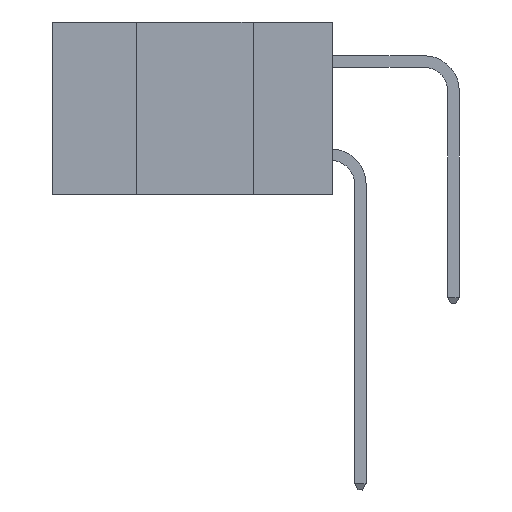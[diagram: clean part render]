
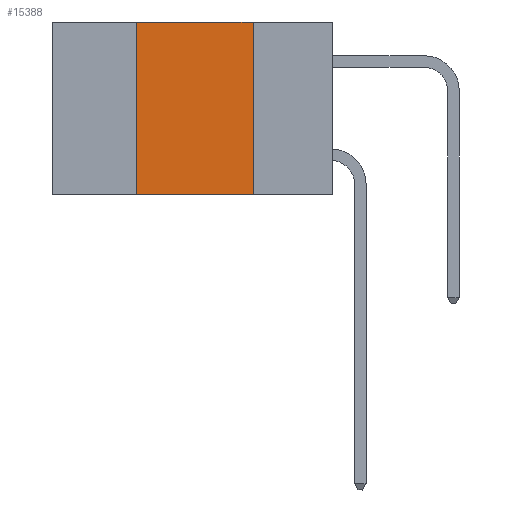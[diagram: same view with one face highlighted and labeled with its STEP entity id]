
A CAD part, left-side view. The second image highlights one B-rep face of the part: STEP entity #15388.
In plain terms, the highlighted planar face has unit normal (-1, 0, 0).
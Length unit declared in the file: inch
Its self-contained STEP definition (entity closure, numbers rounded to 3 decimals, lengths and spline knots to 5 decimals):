
#44 = DIRECTION ( 'NONE',  ( 0., 0., -1. ) ) ;
#180 = EDGE_LOOP ( 'NONE', ( #10132, #4906, #6944, #8728 ) ) ;
#192 = CARTESIAN_POINT ( 'NONE',  ( 0., 0.17, -0.37 ) ) ;
#333 = EDGE_CURVE ( 'NONE', #7812, #22171, #26466, .T. ) ;
#1148 = DIRECTION ( 'NONE',  ( 0., 0., -1. ) ) ;
#3290 = CARTESIAN_POINT ( 'NONE',  ( 0., 0.17, 0. ) ) ;
#4729 = CARTESIAN_POINT ( 'NONE',  ( 0., 0.17, -0.37 ) ) ;
#4906 = ORIENTED_EDGE ( 'NONE', *, *, #18477, .F. ) ;
#6020 = LINE ( 'NONE', #27263, #10728 ) ;
#6132 = DIRECTION ( 'NONE',  ( 0., -1., 0. ) ) ;
#6155 = LINE ( 'NONE', #192, #24782 ) ;
#6944 = ORIENTED_EDGE ( 'NONE', *, *, #333, .F. ) ;
#7812 = VERTEX_POINT ( 'NONE', #26537 ) ;
#8312 = CARTESIAN_POINT ( 'NONE',  ( 0., 0.42, 0. ) ) ;
#8728 = ORIENTED_EDGE ( 'NONE', *, *, #8822, .T. ) ;
#8822 = EDGE_CURVE ( 'NONE', #7812, #20984, #6020, .T. ) ;
#8933 = PLANE ( 'NONE',  #18147 ) ;
#10132 = ORIENTED_EDGE ( 'NONE', *, *, #21232, .F. ) ;
#10728 = VECTOR ( 'NONE', #26968, 39.37008 ) ;
#10842 = DIRECTION ( 'NONE',  ( 0., 0., 1. ) ) ;
#13112 = FACE_OUTER_BOUND ( 'NONE', #180, .T. ) ;
#14755 = CARTESIAN_POINT ( 'NONE',  ( 0., 0.6, 0. ) ) ;
#15388 = ADVANCED_FACE ( 'NONE', ( #13112 ), #8933, .F. ) ;
#17392 = CARTESIAN_POINT ( 'NONE',  ( 0., 0.6, 0. ) ) ;
#18147 = AXIS2_PLACEMENT_3D ( 'NONE', #17392, #23799, #1148 ) ;
#18477 = EDGE_CURVE ( 'NONE', #22171, #27273, #23649, .T. ) ;
#20931 = VECTOR ( 'NONE', #6132, 39.37008 ) ;
#20984 = VERTEX_POINT ( 'NONE', #4729 ) ;
#21232 = EDGE_CURVE ( 'NONE', #27273, #20984, #6155, .T. ) ;
#22155 = CARTESIAN_POINT ( 'NONE',  ( 0., 0.42, -0.37 ) ) ;
#22171 = VERTEX_POINT ( 'NONE', #8312 ) ;
#22928 = VECTOR ( 'NONE', #10842, 39.37008 ) ;
#23649 = LINE ( 'NONE', #14755, #20931 ) ;
#23799 = DIRECTION ( 'NONE',  ( 1., 0., 0. ) ) ;
#24782 = VECTOR ( 'NONE', #44, 39.37008 ) ;
#26466 = LINE ( 'NONE', #22155, #22928 ) ;
#26537 = CARTESIAN_POINT ( 'NONE',  ( 0., 0.42, -0.37 ) ) ;
#26968 = DIRECTION ( 'NONE',  ( 0., -1., 0. ) ) ;
#27263 = CARTESIAN_POINT ( 'NONE',  ( 0., 0.6, -0.37 ) ) ;
#27273 = VERTEX_POINT ( 'NONE', #3290 ) ;
